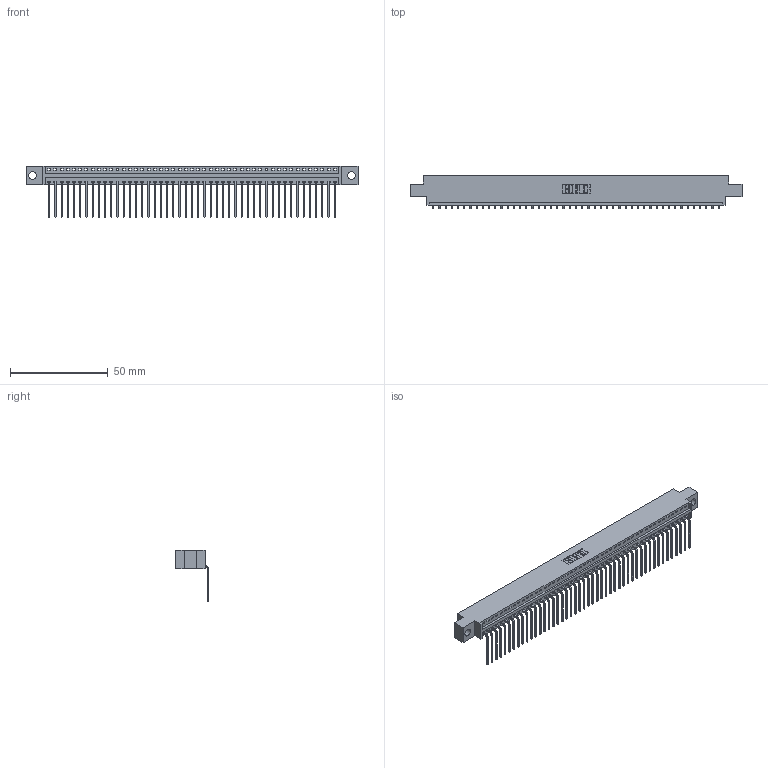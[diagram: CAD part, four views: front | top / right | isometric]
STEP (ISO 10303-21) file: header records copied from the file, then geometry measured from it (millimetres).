
FILE_DESCRIPTION (( 'STEP AP203' ), '1' );
FILE_NAME ('346-047-559-604.STEP', '2022-05-09T22:35:52', ( '' ), ( '' ), 'SwSTEP 2.0', 'SolidWorks 2020', '' );
FILE_SCHEMA (( 'CONFIG_CONTROL_DESIGN' ));
Length unit declared in the file: inch
Products named in the file (3): 345-292-001_558 559 Tail - 1; 346 Part_0.170 Offset - 0.156 Dia-TH; 346-047-559-604
Assembly tree (48 placements, depth 2):
  346-047-559-604
    346 Part_0.170 Offset - 0.156 Dia-TH
    345-292-001_558 559 Tail - 1  x47
Bounding box: 169.8 x 17.08 x 26.16 mm (x, y, z)
Volume: 16184 mm3; surface area: 21213.7 mm2
Topology: 48 solids, 48 shells, 2960 faces, 8931 edges, 5890 vertices
Faces by surface type: plane 2068, cylinder 892
Entity records: 29131 total; most frequent: CARTESIAN_POINT 5003, ORIENTED_EDGE 4982, DIRECTION 4405, EDGE_CURVE 2491, VECTOR 2171, LINE 2171, VERTEX_POINT 1658, AXIS2_PLACEMENT_3D 1117
